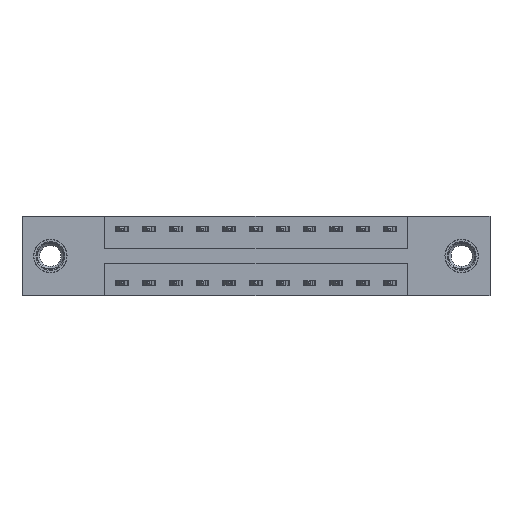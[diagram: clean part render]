
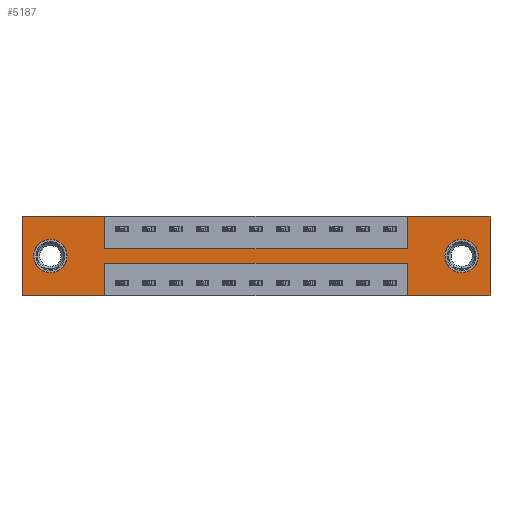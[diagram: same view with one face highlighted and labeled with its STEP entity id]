
A CAD part, front view. The second image highlights one B-rep face of the part: STEP entity #5187.
In plain terms, the highlighted planar face has unit normal (0, -1, 0).
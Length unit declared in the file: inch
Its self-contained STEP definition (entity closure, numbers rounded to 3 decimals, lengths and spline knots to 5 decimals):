
#241 = DIRECTION ( 'NONE',  ( 0., 0., -1. ) ) ;
#278 = CARTESIAN_POINT ( 'NONE',  ( 0.3875, 0., -0.37 ) ) ;
#534 = EDGE_LOOP ( 'NONE', ( #2722, #5818, #3398, #10158, #8524, #10998, #798, #6281, #11274, #9112, #11550, #7176 ) ) ;
#595 = EDGE_LOOP ( 'NONE', ( #6273, #9702 ) ) ;
#610 = AXIS2_PLACEMENT_3D ( 'NONE', #10643, #4888, #11531 ) ;
#798 = ORIENTED_EDGE ( 'NONE', *, *, #4126, .F. ) ;
#920 = CARTESIAN_POINT ( 'NONE',  ( 0., 0., -0.37 ) ) ;
#1013 = EDGE_CURVE ( 'NONE', #2477, #6900, #4720, .T. ) ;
#1104 = CARTESIAN_POINT ( 'NONE',  ( 2.185, 0., 0. ) ) ;
#1191 = CARTESIAN_POINT ( 'NONE',  ( 0., 0., 0. ) ) ;
#1268 = EDGE_CURVE ( 'NONE', #6900, #6845, #11000, .T. ) ;
#1297 = CARTESIAN_POINT ( 'NONE',  ( 1.7975, 0., -0.37 ) ) ;
#1433 = DIRECTION ( 'NONE',  ( 0., 0., 1. ) ) ;
#1532 = VECTOR ( 'NONE', #1433, 39.37008 ) ;
#1613 = EDGE_CURVE ( 'NONE', #3502, #4920, #2080, .T. ) ;
#1677 = EDGE_CURVE ( 'NONE', #11839, #3570, #8810, .T. ) ;
#1750 = VERTEX_POINT ( 'NONE', #10729 ) ;
#1822 = FACE_BOUND ( 'NONE', #4275, .T. ) ;
#1928 = EDGE_CURVE ( 'NONE', #4117, #5397, #3390, .T. ) ;
#2051 = LINE ( 'NONE', #278, #7143 ) ;
#2080 = LINE ( 'NONE', #8635, #7474 ) ;
#2347 = DIRECTION ( 'NONE',  ( 0., 0., 1. ) ) ;
#2398 = EDGE_CURVE ( 'NONE', #4664, #3502, #2051, .T. ) ;
#2437 = CARTESIAN_POINT ( 'NONE',  ( 1.7975, 0., 0. ) ) ;
#2477 = VERTEX_POINT ( 'NONE', #3520 ) ;
#2529 = DIRECTION ( 'NONE',  ( 0., 0., -1. ) ) ;
#2722 = ORIENTED_EDGE ( 'NONE', *, *, #2398, .F. ) ;
#2843 = LINE ( 'NONE', #1297, #7873 ) ;
#3137 = CARTESIAN_POINT ( 'NONE',  ( 0.3875, 0., -0.15 ) ) ;
#3148 = VERTEX_POINT ( 'NONE', #5113 ) ;
#3239 = DIRECTION ( 'NONE',  ( -1., 0., 0. ) ) ;
#3270 = CARTESIAN_POINT ( 'NONE',  ( 0., 0., -0.37 ) ) ;
#3289 = VECTOR ( 'NONE', #11844, 39.37008 ) ;
#3297 = VERTEX_POINT ( 'NONE', #7286 ) ;
#3390 = CIRCLE ( 'NONE', #9089, 0.078 ) ;
#3398 = ORIENTED_EDGE ( 'NONE', *, *, #4017, .F. ) ;
#3435 = EDGE_CURVE ( 'NONE', #6722, #4664, #7104, .T. ) ;
#3473 = CARTESIAN_POINT ( 'NONE',  ( 0., 0., -0.37 ) ) ;
#3502 = VERTEX_POINT ( 'NONE', #11399 ) ;
#3520 = CARTESIAN_POINT ( 'NONE',  ( 2.185, 0., 0. ) ) ;
#3570 = VERTEX_POINT ( 'NONE', #9737 ) ;
#3587 = CARTESIAN_POINT ( 'NONE',  ( 1.7975, 0., -0.22 ) ) ;
#3632 = FACE_BOUND ( 'NONE', #595, .T. ) ;
#3933 = DIRECTION ( 'NONE',  ( 0., 1., 0. ) ) ;
#4005 = LINE ( 'NONE', #3137, #6353 ) ;
#4017 = EDGE_CURVE ( 'NONE', #6845, #6722, #2843, .T. ) ;
#4117 = VERTEX_POINT ( 'NONE', #10347 ) ;
#4126 = EDGE_CURVE ( 'NONE', #3297, #1750, #4324, .T. ) ;
#4130 = EDGE_CURVE ( 'NONE', #10489, #7973, #6952, .T. ) ;
#4239 = VECTOR ( 'NONE', #3239, 39.37008 ) ;
#4275 = EDGE_LOOP ( 'NONE', ( #10007, #10293 ) ) ;
#4324 = LINE ( 'NONE', #2437, #1532 ) ;
#4418 = DIRECTION ( 'NONE',  ( 0., 0., -1. ) ) ;
#4469 = VECTOR ( 'NONE', #12193, 39.37008 ) ;
#4503 = EDGE_CURVE ( 'NONE', #3148, #3297, #4005, .T. ) ;
#4507 = DIRECTION ( 'NONE',  ( 0., -1., 0. ) ) ;
#4657 = CARTESIAN_POINT ( 'NONE',  ( 0.3875, 0., -0.22 ) ) ;
#4662 = CARTESIAN_POINT ( 'NONE',  ( 2.0525, 0., -0.185 ) ) ;
#4664 = VERTEX_POINT ( 'NONE', #6532 ) ;
#4720 = LINE ( 'NONE', #1104, #11958 ) ;
#4888 = DIRECTION ( 'NONE',  ( 0., 1., 0. ) ) ;
#4920 = VERTEX_POINT ( 'NONE', #920 ) ;
#5113 = CARTESIAN_POINT ( 'NONE',  ( 0.3875, 0., -0.15 ) ) ;
#5187 = ADVANCED_FACE ( 'NONE', ( #3632, #1822, #11324 ), #10314, .T. ) ;
#5257 = CARTESIAN_POINT ( 'NONE',  ( 0.3875, 0., 0. ) ) ;
#5397 = VERTEX_POINT ( 'NONE', #5846 ) ;
#5643 = EDGE_CURVE ( 'NONE', #7973, #3148, #10768, .T. ) ;
#5690 = DIRECTION ( 'NONE',  ( 0., 0., -1. ) ) ;
#5818 = ORIENTED_EDGE ( 'NONE', *, *, #3435, .F. ) ;
#5846 = CARTESIAN_POINT ( 'NONE',  ( 2.0525, 0., -0.263 ) ) ;
#5927 = CARTESIAN_POINT ( 'NONE',  ( 0.1325, 0., -0.263 ) ) ;
#6273 = ORIENTED_EDGE ( 'NONE', *, *, #1928, .T. ) ;
#6281 = ORIENTED_EDGE ( 'NONE', *, *, #4503, .F. ) ;
#6353 = VECTOR ( 'NONE', #10925, 39.37008 ) ;
#6363 = DIRECTION ( 'NONE',  ( 0., 1., 0. ) ) ;
#6532 = CARTESIAN_POINT ( 'NONE',  ( 0.3875, 0., -0.22 ) ) ;
#6606 = CARTESIAN_POINT ( 'NONE',  ( 0., 0., 0. ) ) ;
#6722 = VERTEX_POINT ( 'NONE', #3587 ) ;
#6845 = VERTEX_POINT ( 'NONE', #11485 ) ;
#6900 = VERTEX_POINT ( 'NONE', #12404 ) ;
#6952 = LINE ( 'NONE', #7516, #11899 ) ;
#7104 = LINE ( 'NONE', #4657, #4469 ) ;
#7143 = VECTOR ( 'NONE', #4418, 39.37008 ) ;
#7176 = ORIENTED_EDGE ( 'NONE', *, *, #1613, .F. ) ;
#7286 = CARTESIAN_POINT ( 'NONE',  ( 1.7975, 0., -0.15 ) ) ;
#7474 = VECTOR ( 'NONE', #10526, 39.37008 ) ;
#7516 = CARTESIAN_POINT ( 'NONE',  ( 0., 0., 0. ) ) ;
#7585 = DIRECTION ( 'NONE',  ( 1., 0., 0. ) ) ;
#7873 = VECTOR ( 'NONE', #2347, 39.37008 ) ;
#7973 = VERTEX_POINT ( 'NONE', #9353 ) ;
#8190 = EDGE_CURVE ( 'NONE', #3570, #11839, #10853, .T. ) ;
#8480 = DIRECTION ( 'NONE',  ( 1., 0., 0. ) ) ;
#8494 = CARTESIAN_POINT ( 'NONE',  ( 0., 0., 0. ) ) ;
#8524 = ORIENTED_EDGE ( 'NONE', *, *, #1013, .F. ) ;
#8635 = CARTESIAN_POINT ( 'NONE',  ( 0., 0., -0.37 ) ) ;
#8810 = CIRCLE ( 'NONE', #610, 0.078 ) ;
#8935 = VECTOR ( 'NONE', #10162, 39.37008 ) ;
#9089 = AXIS2_PLACEMENT_3D ( 'NONE', #11935, #6363, #241 ) ;
#9112 = ORIENTED_EDGE ( 'NONE', *, *, #4130, .F. ) ;
#9353 = CARTESIAN_POINT ( 'NONE',  ( 0.3875, 0., 0. ) ) ;
#9702 = ORIENTED_EDGE ( 'NONE', *, *, #12576, .T. ) ;
#9737 = CARTESIAN_POINT ( 'NONE',  ( 0.1325, 0., -0.107 ) ) ;
#9770 = CARTESIAN_POINT ( 'NONE',  ( 0.1325, 0., -0.185 ) ) ;
#9834 = VECTOR ( 'NONE', #7585, 39.37008 ) ;
#10007 = ORIENTED_EDGE ( 'NONE', *, *, #8190, .T. ) ;
#10131 = LINE ( 'NONE', #6606, #9834 ) ;
#10158 = ORIENTED_EDGE ( 'NONE', *, *, #1268, .F. ) ;
#10162 = DIRECTION ( 'NONE',  ( 0., 0., 1. ) ) ;
#10202 = EDGE_CURVE ( 'NONE', #4920, #10489, #11373, .T. ) ;
#10293 = ORIENTED_EDGE ( 'NONE', *, *, #1677, .T. ) ;
#10314 = PLANE ( 'NONE',  #11202 ) ;
#10347 = CARTESIAN_POINT ( 'NONE',  ( 2.0525, 0., -0.107 ) ) ;
#10489 = VERTEX_POINT ( 'NONE', #8494 ) ;
#10526 = DIRECTION ( 'NONE',  ( -1., 0., 0. ) ) ;
#10643 = CARTESIAN_POINT ( 'NONE',  ( 0.1325, 0., -0.185 ) ) ;
#10703 = DIRECTION ( 'NONE',  ( 0., 0., 1. ) ) ;
#10729 = CARTESIAN_POINT ( 'NONE',  ( 1.7975, 0., 0. ) ) ;
#10768 = LINE ( 'NONE', #5257, #3289 ) ;
#10793 = AXIS2_PLACEMENT_3D ( 'NONE', #9770, #3933, #10703 ) ;
#10853 = CIRCLE ( 'NONE', #10793, 0.078 ) ;
#10925 = DIRECTION ( 'NONE',  ( 1., 0., 0. ) ) ;
#10998 = ORIENTED_EDGE ( 'NONE', *, *, #12542, .F. ) ;
#11000 = LINE ( 'NONE', #3270, #4239 ) ;
#11202 = AXIS2_PLACEMENT_3D ( 'NONE', #3473, #4507, #11204 ) ;
#11204 = DIRECTION ( 'NONE',  ( 0., 0., -1. ) ) ;
#11274 = ORIENTED_EDGE ( 'NONE', *, *, #5643, .F. ) ;
#11324 = FACE_OUTER_BOUND ( 'NONE', #534, .T. ) ;
#11332 = DIRECTION ( 'NONE',  ( 0., 1., 0. ) ) ;
#11373 = LINE ( 'NONE', #1191, #8935 ) ;
#11399 = CARTESIAN_POINT ( 'NONE',  ( 0.3875, 0., -0.37 ) ) ;
#11485 = CARTESIAN_POINT ( 'NONE',  ( 1.7975, 0., -0.37 ) ) ;
#11531 = DIRECTION ( 'NONE',  ( 0., 0., 1. ) ) ;
#11550 = ORIENTED_EDGE ( 'NONE', *, *, #10202, .F. ) ;
#11839 = VERTEX_POINT ( 'NONE', #5927 ) ;
#11844 = DIRECTION ( 'NONE',  ( 0., 0., -1. ) ) ;
#11899 = VECTOR ( 'NONE', #8480, 39.37008 ) ;
#11935 = CARTESIAN_POINT ( 'NONE',  ( 2.0525, 0., -0.185 ) ) ;
#11958 = VECTOR ( 'NONE', #2529, 39.37008 ) ;
#12189 = CIRCLE ( 'NONE', #12561, 0.078 ) ;
#12193 = DIRECTION ( 'NONE',  ( -1., 0., 0. ) ) ;
#12404 = CARTESIAN_POINT ( 'NONE',  ( 2.185, 0., -0.37 ) ) ;
#12542 = EDGE_CURVE ( 'NONE', #1750, #2477, #10131, .T. ) ;
#12561 = AXIS2_PLACEMENT_3D ( 'NONE', #4662, #11332, #5690 ) ;
#12576 = EDGE_CURVE ( 'NONE', #5397, #4117, #12189, .T. ) ;
